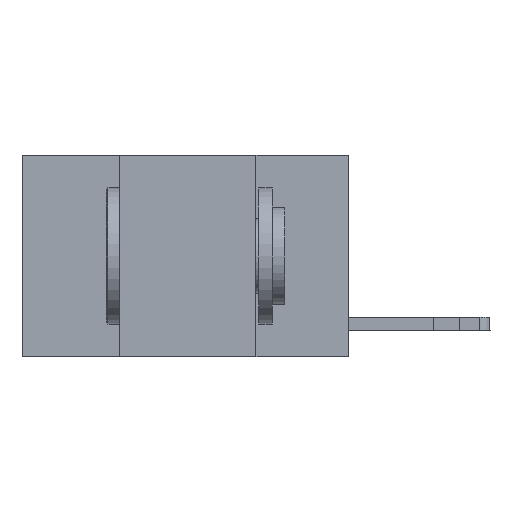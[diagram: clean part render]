
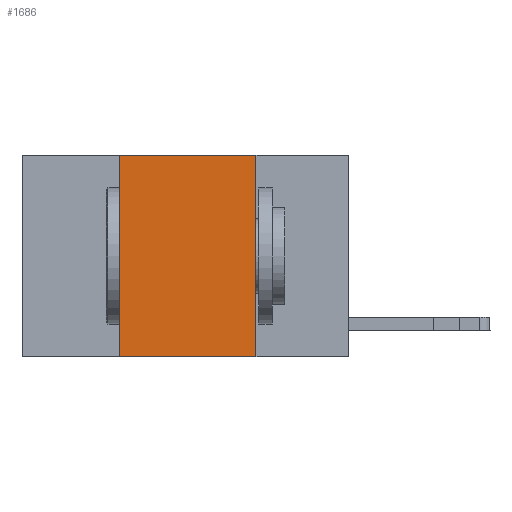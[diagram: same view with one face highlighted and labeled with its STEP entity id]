
A CAD part, left-side view. The second image highlights one B-rep face of the part: STEP entity #1686.
In plain terms, the highlighted planar face has unit normal (-1, 0, 0).
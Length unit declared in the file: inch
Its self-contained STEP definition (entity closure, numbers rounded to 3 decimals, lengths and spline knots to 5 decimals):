
#115 = ORIENTED_EDGE ( 'NONE', *, *, #13908, .T. ) ;
#178 = EDGE_CURVE ( 'NONE', #7906, #6195, #10655, .T. ) ;
#532 = ORIENTED_EDGE ( 'NONE', *, *, #14705, .F. ) ;
#763 = DIRECTION ( 'NONE',  ( 0., -1., 0. ) ) ;
#1322 = VERTEX_POINT ( 'NONE', #11886 ) ;
#1382 = EDGE_CURVE ( 'NONE', #1322, #7906, #10945, .T. ) ;
#1686 = ADVANCED_FACE ( 'NONE', ( #3202 ), #13697, .F. ) ;
#3202 = FACE_OUTER_BOUND ( 'NONE', #12406, .T. ) ;
#4034 = VECTOR ( 'NONE', #5361, 39.37008 ) ;
#4048 = DIRECTION ( 'NONE',  ( 1., 0., 0. ) ) ;
#4804 = CARTESIAN_POINT ( 'NONE',  ( 0., 0.42, 0. ) ) ;
#5361 = DIRECTION ( 'NONE',  ( 0., 0., -1. ) ) ;
#5803 = CARTESIAN_POINT ( 'NONE',  ( 0., 0.6, 0. ) ) ;
#5907 = CARTESIAN_POINT ( 'NONE',  ( 0., 0.17, 0. ) ) ;
#6030 = DIRECTION ( 'NONE',  ( 0., 0., 1. ) ) ;
#6038 = VECTOR ( 'NONE', #763, 39.37008 ) ;
#6195 = VERTEX_POINT ( 'NONE', #7128 ) ;
#6401 = LINE ( 'NONE', #4804, #12645 ) ;
#7128 = CARTESIAN_POINT ( 'NONE',  ( 0., 0.17, -0.37 ) ) ;
#7413 = CARTESIAN_POINT ( 'NONE',  ( 0., 0.42, -0.37 ) ) ;
#7564 = CARTESIAN_POINT ( 'NONE',  ( 0., 0.6, 0. ) ) ;
#7906 = VERTEX_POINT ( 'NONE', #8050 ) ;
#8050 = CARTESIAN_POINT ( 'NONE',  ( 0., 0.17, 0. ) ) ;
#8204 = VERTEX_POINT ( 'NONE', #7413 ) ;
#8406 = ORIENTED_EDGE ( 'NONE', *, *, #178, .F. ) ;
#9023 = LINE ( 'NONE', #15619, #6038 ) ;
#9797 = AXIS2_PLACEMENT_3D ( 'NONE', #5803, #4048, #11236 ) ;
#10655 = LINE ( 'NONE', #5907, #4034 ) ;
#10945 = LINE ( 'NONE', #7564, #12931 ) ;
#11236 = DIRECTION ( 'NONE',  ( 0., 0., -1. ) ) ;
#11886 = CARTESIAN_POINT ( 'NONE',  ( 0., 0.42, 0. ) ) ;
#12406 = EDGE_LOOP ( 'NONE', ( #8406, #14570, #532, #115 ) ) ;
#12645 = VECTOR ( 'NONE', #6030, 39.37008 ) ;
#12931 = VECTOR ( 'NONE', #15946, 39.37008 ) ;
#13697 = PLANE ( 'NONE',  #9797 ) ;
#13908 = EDGE_CURVE ( 'NONE', #8204, #6195, #9023, .T. ) ;
#14570 = ORIENTED_EDGE ( 'NONE', *, *, #1382, .F. ) ;
#14705 = EDGE_CURVE ( 'NONE', #8204, #1322, #6401, .T. ) ;
#15619 = CARTESIAN_POINT ( 'NONE',  ( 0., 0.6, -0.37 ) ) ;
#15946 = DIRECTION ( 'NONE',  ( 0., -1., 0. ) ) ;
